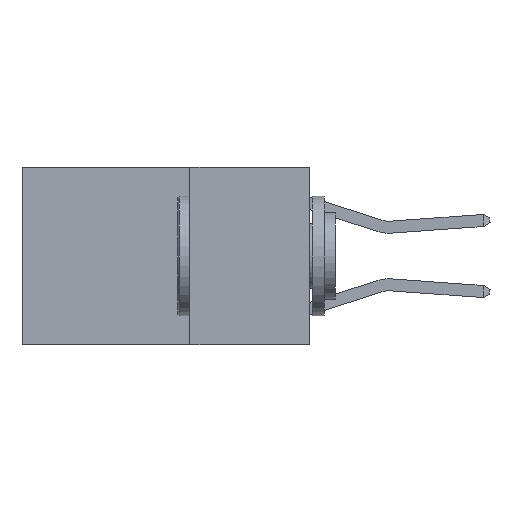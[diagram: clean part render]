
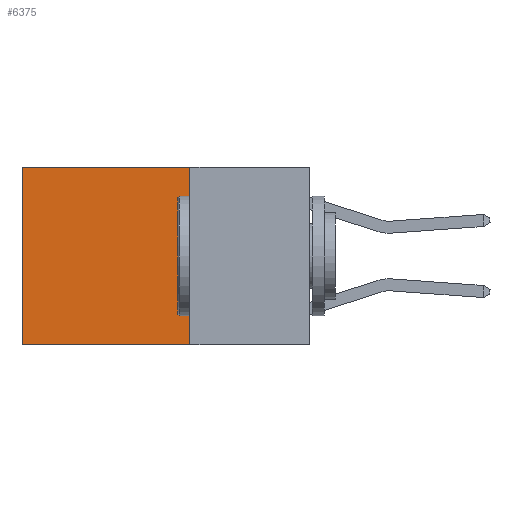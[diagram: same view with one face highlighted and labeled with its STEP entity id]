
A CAD part, left-side view. The second image highlights one B-rep face of the part: STEP entity #6375.
In plain terms, the highlighted planar face has unit normal (-1, 0, 0).
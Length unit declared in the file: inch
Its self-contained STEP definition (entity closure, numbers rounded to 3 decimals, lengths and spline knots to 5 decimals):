
#182 = VECTOR ( 'NONE', #11471, 39.37008 ) ;
#491 = DIRECTION ( 'NONE',  ( 0., 0., -1. ) ) ;
#1018 = VERTEX_POINT ( 'NONE', #3284 ) ;
#1536 = LINE ( 'NONE', #6468, #2406 ) ;
#1790 = EDGE_CURVE ( 'NONE', #1018, #7488, #1536, .T. ) ;
#2406 = VECTOR ( 'NONE', #9652, 39.37008 ) ;
#2933 = ORIENTED_EDGE ( 'NONE', *, *, #3222, .F. ) ;
#3222 = EDGE_CURVE ( 'NONE', #3271, #1018, #12309, .T. ) ;
#3271 = VERTEX_POINT ( 'NONE', #3570 ) ;
#3284 = CARTESIAN_POINT ( 'NONE',  ( 0.2625, 0.25, -0.37 ) ) ;
#3427 = PLANE ( 'NONE',  #8281 ) ;
#3477 = CARTESIAN_POINT ( 'NONE',  ( 0.2625, 0.6, 0. ) ) ;
#3570 = CARTESIAN_POINT ( 'NONE',  ( 0.2625, 0.25, 0. ) ) ;
#3779 = CARTESIAN_POINT ( 'NONE',  ( 0.2625, 0.6, 0. ) ) ;
#3884 = ORIENTED_EDGE ( 'NONE', *, *, #1790, .F. ) ;
#4166 = CARTESIAN_POINT ( 'NONE',  ( 0.2625, 0.25, 0. ) ) ;
#4194 = ORIENTED_EDGE ( 'NONE', *, *, #6623, .T. ) ;
#4619 = CARTESIAN_POINT ( 'NONE',  ( 0.2625, 0.6, -0.37 ) ) ;
#5486 = ORIENTED_EDGE ( 'NONE', *, *, #10130, .T. ) ;
#6055 = VERTEX_POINT ( 'NONE', #3779 ) ;
#6116 = VECTOR ( 'NONE', #10171, 39.37008 ) ;
#6375 = ADVANCED_FACE ( 'NONE', ( #10132 ), #3427, .F. ) ;
#6437 = VECTOR ( 'NONE', #11757, 39.37008 ) ;
#6468 = CARTESIAN_POINT ( 'NONE',  ( 0.2625, 0.25, -0.37 ) ) ;
#6623 = EDGE_CURVE ( 'NONE', #6055, #7488, #7213, .T. ) ;
#7213 = LINE ( 'NONE', #3477, #6116 ) ;
#7488 = VERTEX_POINT ( 'NONE', #4619 ) ;
#7521 = CARTESIAN_POINT ( 'NONE',  ( 0.2625, 0.25, 0. ) ) ;
#8011 = LINE ( 'NONE', #4166, #6437 ) ;
#8106 = CARTESIAN_POINT ( 'NONE',  ( 0.2625, 0.25, 0. ) ) ;
#8223 = DIRECTION ( 'NONE',  ( 1., 0., 0. ) ) ;
#8281 = AXIS2_PLACEMENT_3D ( 'NONE', #8106, #8223, #491 ) ;
#9652 = DIRECTION ( 'NONE',  ( 0., 1., 0. ) ) ;
#10130 = EDGE_CURVE ( 'NONE', #3271, #6055, #8011, .T. ) ;
#10132 = FACE_OUTER_BOUND ( 'NONE', #12159, .T. ) ;
#10171 = DIRECTION ( 'NONE',  ( 0., 0., -1. ) ) ;
#11471 = DIRECTION ( 'NONE',  ( 0., 0., -1. ) ) ;
#11757 = DIRECTION ( 'NONE',  ( 0., 1., 0. ) ) ;
#12159 = EDGE_LOOP ( 'NONE', ( #4194, #3884, #2933, #5486 ) ) ;
#12309 = LINE ( 'NONE', #7521, #182 ) ;
